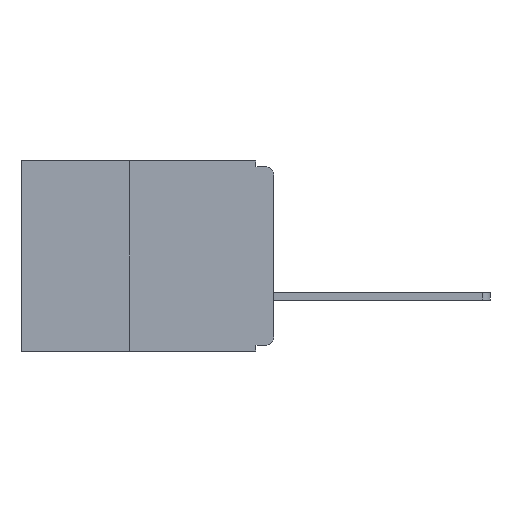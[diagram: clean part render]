
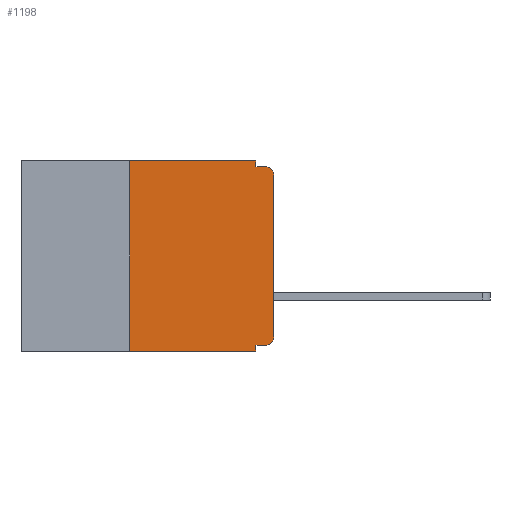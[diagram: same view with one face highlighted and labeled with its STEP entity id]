
A CAD part, left-side view. The second image highlights one B-rep face of the part: STEP entity #1198.
In plain terms, the highlighted planar face has unit normal (-1, 0, 0).
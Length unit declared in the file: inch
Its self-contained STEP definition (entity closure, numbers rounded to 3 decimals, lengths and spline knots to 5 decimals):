
#321 = ORIENTED_EDGE ( 'NONE', *, *, #11447, .F. ) ;
#333 = VECTOR ( 'NONE', #8773, 39.37008 ) ;
#433 = LINE ( 'NONE', #9013, #333 ) ;
#577 = CARTESIAN_POINT ( 'NONE',  ( 0., 0.031, -0.33 ) ) ;
#633 = VECTOR ( 'NONE', #13244, 39.37008 ) ;
#674 = AXIS2_PLACEMENT_3D ( 'NONE', #8624, #8489, #8443 ) ;
#778 = ORIENTED_EDGE ( 'NONE', *, *, #1279, .F. ) ;
#926 = LINE ( 'NONE', #13114, #633 ) ;
#970 = ORIENTED_EDGE ( 'NONE', *, *, #3686, .F. ) ;
#1198 = ADVANCED_FACE ( 'NONE', ( #3087 ), #9591, .F. ) ;
#1213 = VECTOR ( 'NONE', #10923, 39.37008 ) ;
#1279 = EDGE_CURVE ( 'NONE', #2069, #3602, #1759, .T. ) ;
#1302 = LINE ( 'NONE', #11944, #1213 ) ;
#1307 = CARTESIAN_POINT ( 'NONE',  ( 0., 0., -0.305 ) ) ;
#1310 = EDGE_CURVE ( 'NONE', #10024, #1546, #1302, .T. ) ;
#1312 = EDGE_CURVE ( 'NONE', #10024, #6890, #926, .T. ) ;
#1344 = EDGE_CURVE ( 'NONE', #7781, #6890, #433, .T. ) ;
#1352 = VECTOR ( 'NONE', #17221, 39.37008 ) ;
#1422 = EDGE_CURVE ( 'NONE', #1722, #1543, #18585, .T. ) ;
#1487 = CARTESIAN_POINT ( 'NONE',  ( 0., 0.031, 0. ) ) ;
#1543 = VERTEX_POINT ( 'NONE', #14013 ) ;
#1546 = VERTEX_POINT ( 'NONE', #13793 ) ;
#1722 = VERTEX_POINT ( 'NONE', #5276 ) ;
#1751 = ORIENTED_EDGE ( 'NONE', *, *, #1310, .F. ) ;
#1759 = LINE ( 'NONE', #1487, #1352 ) ;
#2000 = AXIS2_PLACEMENT_3D ( 'NONE', #7956, #7161, #7036 ) ;
#2069 = VERTEX_POINT ( 'NONE', #12948 ) ;
#2295 = VERTEX_POINT ( 'NONE', #18885 ) ;
#2871 = VECTOR ( 'NONE', #7166, 39.37008 ) ;
#2986 = LINE ( 'NONE', #6644, #2871 ) ;
#3087 = FACE_OUTER_BOUND ( 'NONE', #9105, .T. ) ;
#3419 = ORIENTED_EDGE ( 'NONE', *, *, #1312, .T. ) ;
#3602 = VERTEX_POINT ( 'NONE', #9351 ) ;
#3686 = EDGE_CURVE ( 'NONE', #1546, #2069, #7814, .T. ) ;
#4945 = ORIENTED_EDGE ( 'NONE', *, *, #16675, .T. ) ;
#5276 = CARTESIAN_POINT ( 'NONE',  ( 0., 0., -0.025 ) ) ;
#6028 = VECTOR ( 'NONE', #11711, 39.37008 ) ;
#6321 = EDGE_CURVE ( 'NONE', #2295, #7781, #6580, .T. ) ;
#6580 = LINE ( 'NONE', #11976, #6028 ) ;
#6644 = CARTESIAN_POINT ( 'NONE',  ( 0., 0., -0.01 ) ) ;
#6890 = VERTEX_POINT ( 'NONE', #577 ) ;
#6936 = ORIENTED_EDGE ( 'NONE', *, *, #1344, .F. ) ;
#7036 = DIRECTION ( 'NONE',  ( 0., 0., -1. ) ) ;
#7158 = DIRECTION ( 'NONE',  ( 0., -1., 0. ) ) ;
#7161 = DIRECTION ( 'NONE',  ( 1., 0., 0. ) ) ;
#7166 = DIRECTION ( 'NONE',  ( 0., -1., 0. ) ) ;
#7555 = CARTESIAN_POINT ( 'NONE',  ( 0., 0.437, 0. ) ) ;
#7781 = VERTEX_POINT ( 'NONE', #16804 ) ;
#7797 = VECTOR ( 'NONE', #7158, 39.37008 ) ;
#7814 = LINE ( 'NONE', #7555, #7797 ) ;
#7956 = CARTESIAN_POINT ( 'NONE',  ( 0., 0.437, 0. ) ) ;
#8443 = DIRECTION ( 'NONE',  ( 0., 0., -1. ) ) ;
#8489 = DIRECTION ( 'NONE',  ( -1., 0., 0. ) ) ;
#8624 = CARTESIAN_POINT ( 'NONE',  ( 0., 0.015, -0.305 ) ) ;
#8676 = VERTEX_POINT ( 'NONE', #1307 ) ;
#8773 = DIRECTION ( 'NONE',  ( 0., 0., -1. ) ) ;
#9013 = CARTESIAN_POINT ( 'NONE',  ( 0., 0.031, -0.33 ) ) ;
#9105 = EDGE_LOOP ( 'NONE', ( #4945, #18078, #321, #778, #970, #1751, #3419, #6936, #10389, #11700 ) ) ;
#9351 = CARTESIAN_POINT ( 'NONE',  ( 0., 0.031, -0.01 ) ) ;
#9591 = PLANE ( 'NONE',  #2000 ) ;
#10024 = VERTEX_POINT ( 'NONE', #16034 ) ;
#10389 = ORIENTED_EDGE ( 'NONE', *, *, #6321, .F. ) ;
#10589 = LINE ( 'NONE', #11695, #10606 ) ;
#10606 = VECTOR ( 'NONE', #11727, 39.37008 ) ;
#10923 = DIRECTION ( 'NONE',  ( 0., 0., 1. ) ) ;
#11447 = EDGE_CURVE ( 'NONE', #3602, #1543, #2986, .T. ) ;
#11695 = CARTESIAN_POINT ( 'NONE',  ( 0., 0., 0. ) ) ;
#11700 = ORIENTED_EDGE ( 'NONE', *, *, #13746, .T. ) ;
#11711 = DIRECTION ( 'NONE',  ( 0., 1., 0. ) ) ;
#11727 = DIRECTION ( 'NONE',  ( 0., 0., 1. ) ) ;
#11944 = CARTESIAN_POINT ( 'NONE',  ( 0., 0.25, -0.33 ) ) ;
#11976 = CARTESIAN_POINT ( 'NONE',  ( 0., 0., -0.32 ) ) ;
#12852 = AXIS2_PLACEMENT_3D ( 'NONE', #18146, #18126, #18093 ) ;
#12948 = CARTESIAN_POINT ( 'NONE',  ( 0., 0.031, 0. ) ) ;
#13027 = CIRCLE ( 'NONE', #674, 0.015 ) ;
#13114 = CARTESIAN_POINT ( 'NONE',  ( 0., 0.437, -0.33 ) ) ;
#13244 = DIRECTION ( 'NONE',  ( 0., -1., 0. ) ) ;
#13746 = EDGE_CURVE ( 'NONE', #2295, #8676, #13027, .T. ) ;
#13793 = CARTESIAN_POINT ( 'NONE',  ( 0., 0.25, 0. ) ) ;
#14013 = CARTESIAN_POINT ( 'NONE',  ( 0., 0.015, -0.01 ) ) ;
#16034 = CARTESIAN_POINT ( 'NONE',  ( 0., 0.25, -0.33 ) ) ;
#16675 = EDGE_CURVE ( 'NONE', #8676, #1722, #10589, .T. ) ;
#16804 = CARTESIAN_POINT ( 'NONE',  ( 0., 0.031, -0.32 ) ) ;
#17221 = DIRECTION ( 'NONE',  ( 0., 0., -1. ) ) ;
#18078 = ORIENTED_EDGE ( 'NONE', *, *, #1422, .T. ) ;
#18093 = DIRECTION ( 'NONE',  ( 0., 0., -1. ) ) ;
#18126 = DIRECTION ( 'NONE',  ( -1., 0., 0. ) ) ;
#18146 = CARTESIAN_POINT ( 'NONE',  ( 0., 0.015, -0.025 ) ) ;
#18585 = CIRCLE ( 'NONE', #12852, 0.015 ) ;
#18885 = CARTESIAN_POINT ( 'NONE',  ( 0., 0.015, -0.32 ) ) ;
